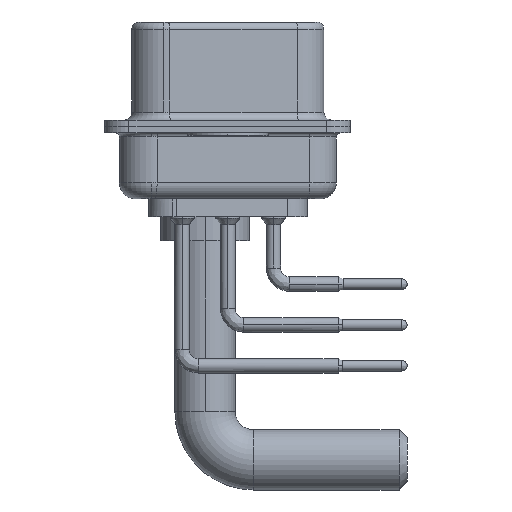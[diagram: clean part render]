
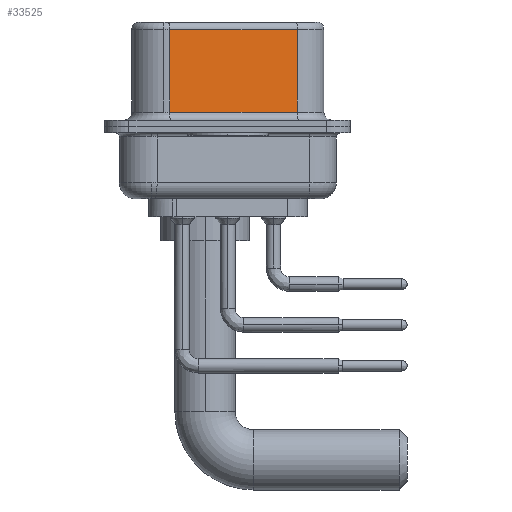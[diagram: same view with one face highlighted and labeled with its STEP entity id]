
A CAD part, left-side view. The second image highlights one B-rep face of the part: STEP entity #33525.
In plain terms, the highlighted planar face has unit normal (-0.985, -0.174, 0).
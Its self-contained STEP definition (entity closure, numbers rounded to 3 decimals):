
#3064 = PLANE ( 'NONE',  #6405 ) ;
#4097 = ORIENTED_EDGE ( 'NONE', *, *, #33588, .F. ) ;
#4273 = ORIENTED_EDGE ( 'NONE', *, *, #18174, .T. ) ;
#4659 = VERTEX_POINT ( 'NONE', #15977 ) ;
#5323 = LINE ( 'NONE', #21160, #28575 ) ;
#5505 = DIRECTION ( 'NONE',  ( 0.985, 0.174, 0. ) ) ;
#6405 = AXIS2_PLACEMENT_3D ( 'NONE', #27249, #5505, #14224 ) ;
#7246 = DIRECTION ( 'NONE',  ( -0.174, 0.985, 0. ) ) ;
#7596 = LINE ( 'NONE', #20473, #31525 ) ;
#7663 = ORIENTED_EDGE ( 'NONE', *, *, #22064, .T. ) ;
#8286 = CARTESIAN_POINT ( 'NONE',  ( 5.132, -4.322, 6.52 ) ) ;
#10057 = ORIENTED_EDGE ( 'NONE', *, *, #30071, .T. ) ;
#10441 = CARTESIAN_POINT ( 'NONE',  ( 5.132, -4.322, 0.9 ) ) ;
#11208 = VECTOR ( 'NONE', #27657, 1000. ) ;
#13332 = DIRECTION ( 'NONE',  ( 0., 0., -1. ) ) ;
#14224 = DIRECTION ( 'NONE',  ( -0.174, 0.985, 0. ) ) ;
#14240 = VERTEX_POINT ( 'NONE', #18807 ) ;
#14285 = CARTESIAN_POINT ( 'NONE',  ( 5.132, -4.322, 0.9 ) ) ;
#14648 = VERTEX_POINT ( 'NONE', #10441 ) ;
#15977 = CARTESIAN_POINT ( 'NONE',  ( 5.132, -4.322, 6.02 ) ) ;
#16558 = EDGE_LOOP ( 'NONE', ( #4097, #7663, #4273, #10057 ) ) ;
#18174 = EDGE_CURVE ( 'NONE', #30391, #14240, #5323, .T. ) ;
#18616 = VECTOR ( 'NONE', #18889, 1000. ) ;
#18807 = CARTESIAN_POINT ( 'NONE',  ( 3.73, 3.628, 0.9 ) ) ;
#18889 = DIRECTION ( 'NONE',  ( 0., 0., -1. ) ) ;
#20071 = CARTESIAN_POINT ( 'NONE',  ( 3.73, 3.628, 6.02 ) ) ;
#20473 = CARTESIAN_POINT ( 'NONE',  ( 5.132, -4.322, 6.02 ) ) ;
#21160 = CARTESIAN_POINT ( 'NONE',  ( 3.73, 3.628, 6.52 ) ) ;
#22064 = EDGE_CURVE ( 'NONE', #4659, #30391, #7596, .T. ) ;
#27249 = CARTESIAN_POINT ( 'NONE',  ( 5.132, -4.322, 6.52 ) ) ;
#27657 = DIRECTION ( 'NONE',  ( 0.174, -0.985, 0. ) ) ;
#28575 = VECTOR ( 'NONE', #13332, 1000. ) ;
#29348 = FACE_OUTER_BOUND ( 'NONE', #16558, .T. ) ;
#30071 = EDGE_CURVE ( 'NONE', #14240, #14648, #30276, .T. ) ;
#30276 = LINE ( 'NONE', #14285, #11208 ) ;
#30391 = VERTEX_POINT ( 'NONE', #20071 ) ;
#31525 = VECTOR ( 'NONE', #7246, 1000. ) ;
#32137 = LINE ( 'NONE', #8286, #18616 ) ;
#33525 = ADVANCED_FACE ( 'NONE', ( #29348 ), #3064, .F. ) ;
#33588 = EDGE_CURVE ( 'NONE', #4659, #14648, #32137, .T. ) ;
